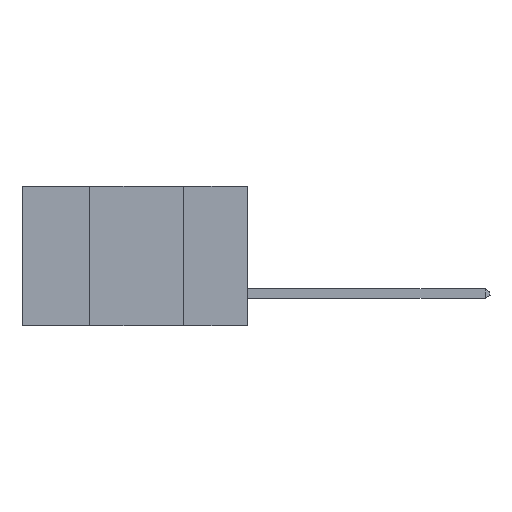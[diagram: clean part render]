
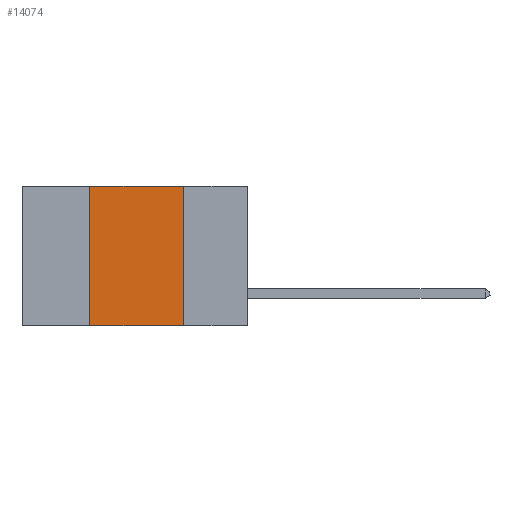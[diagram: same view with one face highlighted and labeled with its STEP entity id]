
A CAD part, left-side view. The second image highlights one B-rep face of the part: STEP entity #14074.
In plain terms, the highlighted planar face has unit normal (-1, 0, 0).
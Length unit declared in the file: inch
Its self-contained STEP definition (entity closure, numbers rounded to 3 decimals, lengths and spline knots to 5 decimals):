
#102 = DIRECTION ( 'NONE',  ( 0., 0., 1. ) ) ;
#866 = ORIENTED_EDGE ( 'NONE', *, *, #1886, .F. ) ;
#1208 = ORIENTED_EDGE ( 'NONE', *, *, #10865, .F. ) ;
#1886 = EDGE_CURVE ( 'NONE', #3217, #9269, #11123, .T. ) ;
#2075 = FACE_OUTER_BOUND ( 'NONE', #6313, .T. ) ;
#2698 = EDGE_CURVE ( 'NONE', #3217, #3551, #15939, .T. ) ;
#2840 = DIRECTION ( 'NONE',  ( 0., -1., 0. ) ) ;
#3041 = CARTESIAN_POINT ( 'NONE',  ( 0., 0.42, 0. ) ) ;
#3217 = VERTEX_POINT ( 'NONE', #4414 ) ;
#3551 = VERTEX_POINT ( 'NONE', #6088 ) ;
#3662 = VECTOR ( 'NONE', #2840, 39.37008 ) ;
#4414 = CARTESIAN_POINT ( 'NONE',  ( 0., 0.42, -0.37 ) ) ;
#4816 = LINE ( 'NONE', #11748, #14064 ) ;
#5286 = VECTOR ( 'NONE', #8855, 39.37008 ) ;
#5567 = DIRECTION ( 'NONE',  ( 0., -1., 0. ) ) ;
#6088 = CARTESIAN_POINT ( 'NONE',  ( 0., 0.17, -0.37 ) ) ;
#6110 = AXIS2_PLACEMENT_3D ( 'NONE', #9648, #9484, #15996 ) ;
#6313 = EDGE_LOOP ( 'NONE', ( #1208, #11950, #866, #15670 ) ) ;
#7220 = CARTESIAN_POINT ( 'NONE',  ( 0., 0.17, 0. ) ) ;
#7743 = CARTESIAN_POINT ( 'NONE',  ( 0., 0.42, 0. ) ) ;
#8788 = VERTEX_POINT ( 'NONE', #11203 ) ;
#8855 = DIRECTION ( 'NONE',  ( 0., 0., -1. ) ) ;
#9269 = VERTEX_POINT ( 'NONE', #3041 ) ;
#9484 = DIRECTION ( 'NONE',  ( 1., 0., 0. ) ) ;
#9648 = CARTESIAN_POINT ( 'NONE',  ( 0., 0.6, 0. ) ) ;
#10517 = CARTESIAN_POINT ( 'NONE',  ( 0., 0.6, -0.37 ) ) ;
#10865 = EDGE_CURVE ( 'NONE', #8788, #3551, #12126, .T. ) ;
#11123 = LINE ( 'NONE', #7743, #16595 ) ;
#11203 = CARTESIAN_POINT ( 'NONE',  ( 0., 0.17, 0. ) ) ;
#11748 = CARTESIAN_POINT ( 'NONE',  ( 0., 0.6, 0. ) ) ;
#11950 = ORIENTED_EDGE ( 'NONE', *, *, #12400, .F. ) ;
#12126 = LINE ( 'NONE', #7220, #5286 ) ;
#12135 = PLANE ( 'NONE',  #6110 ) ;
#12400 = EDGE_CURVE ( 'NONE', #9269, #8788, #4816, .T. ) ;
#14064 = VECTOR ( 'NONE', #5567, 39.37008 ) ;
#14074 = ADVANCED_FACE ( 'NONE', ( #2075 ), #12135, .F. ) ;
#15670 = ORIENTED_EDGE ( 'NONE', *, *, #2698, .T. ) ;
#15939 = LINE ( 'NONE', #10517, #3662 ) ;
#15996 = DIRECTION ( 'NONE',  ( 0., 0., -1. ) ) ;
#16595 = VECTOR ( 'NONE', #102, 39.37008 ) ;
